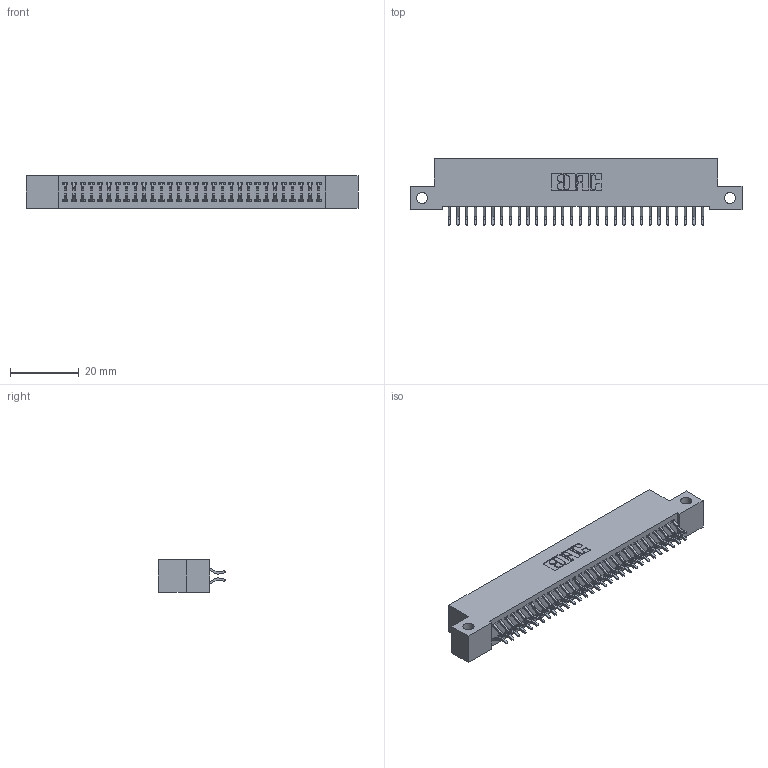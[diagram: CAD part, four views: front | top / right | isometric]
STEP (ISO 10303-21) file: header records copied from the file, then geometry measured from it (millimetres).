
FILE_DESCRIPTION (( 'STEP AP203' ), '1' );
FILE_NAME ('342-060-556-212.STEP', '2019-10-03T13:34:06', ( '' ), ( '' ), 'SwSTEP 2.0', 'SolidWorks 2016', '' );
FILE_SCHEMA (( 'CONFIG_CONTROL_DESIGN' ));
Length unit declared in the file: inch
Products named in the file (3): 342 Part_Side Mount; 345-292-001_556 Tail; 342-060-556-212
Assembly tree (61 placements, depth 2):
  342-060-556-212
    342 Part_Side Mount
    345-292-001_556 Tail  x60
Bounding box: 96.52 x 19.58 x 9.4 mm (x, y, z)
Volume: 8540.1 mm3; surface area: 13387.4 mm2
Topology: 61 solids, 61 shells, 3590 faces, 10679 edges, 7038 vertices
Faces by surface type: plane 2466, cylinder 1124
Entity records: 20943 total; most frequent: CARTESIAN_POINT 3498, ORIENTED_EDGE 3422, DIRECTION 2999, EDGE_CURVE 1711, VECTOR 1575, LINE 1575, VERTEX_POINT 1138, AXIS2_PLACEMENT_3D 712
